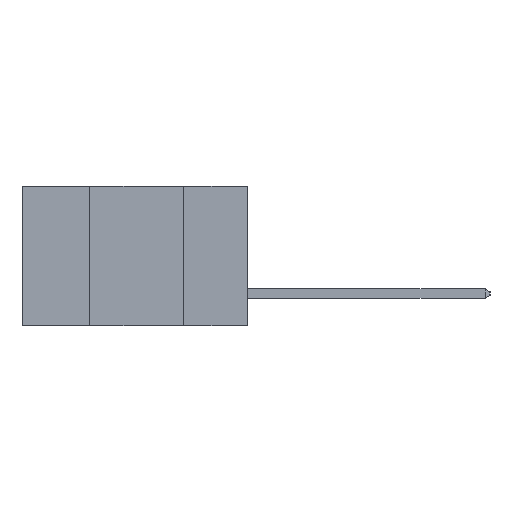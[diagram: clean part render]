
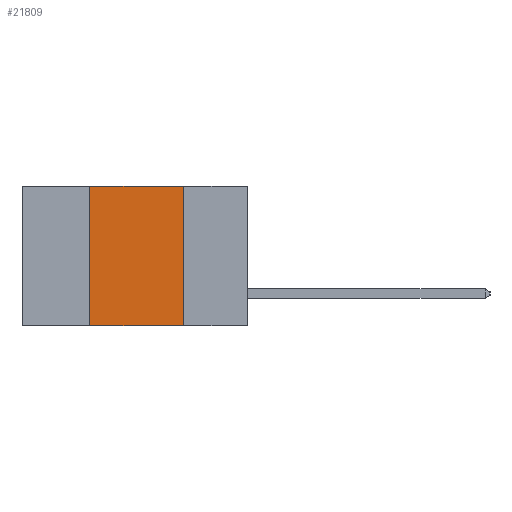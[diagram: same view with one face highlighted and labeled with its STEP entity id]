
A CAD part, left-side view. The second image highlights one B-rep face of the part: STEP entity #21809.
In plain terms, the highlighted planar face has unit normal (-1, 0, 0).
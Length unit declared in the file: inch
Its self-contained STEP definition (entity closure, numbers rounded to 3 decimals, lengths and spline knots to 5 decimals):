
#1304 = CARTESIAN_POINT ( 'NONE',  ( 0., 0.42, -0.37 ) ) ;
#1460 = CARTESIAN_POINT ( 'NONE',  ( 0., 0.17, 0. ) ) ;
#2039 = EDGE_CURVE ( 'NONE', #16251, #20413, #9631, .T. ) ;
#2403 = CARTESIAN_POINT ( 'NONE',  ( 0., 0.42, 0. ) ) ;
#2619 = CARTESIAN_POINT ( 'NONE',  ( 0., 0.6, 0. ) ) ;
#2816 = CARTESIAN_POINT ( 'NONE',  ( 0., 0.42, 0. ) ) ;
#4163 = VECTOR ( 'NONE', #11930, 39.37008 ) ;
#4676 = DIRECTION ( 'NONE',  ( 1., 0., 0. ) ) ;
#5039 = VERTEX_POINT ( 'NONE', #1304 ) ;
#5864 = LINE ( 'NONE', #18044, #25113 ) ;
#5946 = EDGE_CURVE ( 'NONE', #20413, #9562, #23006, .T. ) ;
#6793 = ORIENTED_EDGE ( 'NONE', *, *, #18635, .F. ) ;
#6980 = CARTESIAN_POINT ( 'NONE',  ( 0., 0.17, -0.37 ) ) ;
#6997 = DIRECTION ( 'NONE',  ( 0., 0., -1. ) ) ;
#8268 = AXIS2_PLACEMENT_3D ( 'NONE', #2619, #4676, #18788 ) ;
#9192 = EDGE_LOOP ( 'NONE', ( #21666, #16491, #6793, #16978 ) ) ;
#9562 = VERTEX_POINT ( 'NONE', #6980 ) ;
#9631 = LINE ( 'NONE', #11522, #4163 ) ;
#11522 = CARTESIAN_POINT ( 'NONE',  ( 0., 0.6, 0. ) ) ;
#11930 = DIRECTION ( 'NONE',  ( 0., -1., 0. ) ) ;
#13063 = LINE ( 'NONE', #2403, #18353 ) ;
#14804 = PLANE ( 'NONE',  #8268 ) ;
#15982 = EDGE_CURVE ( 'NONE', #5039, #9562, #5864, .T. ) ;
#16251 = VERTEX_POINT ( 'NONE', #2816 ) ;
#16491 = ORIENTED_EDGE ( 'NONE', *, *, #2039, .F. ) ;
#16978 = ORIENTED_EDGE ( 'NONE', *, *, #15982, .T. ) ;
#17901 = VECTOR ( 'NONE', #6997, 39.37008 ) ;
#18044 = CARTESIAN_POINT ( 'NONE',  ( 0., 0.6, -0.37 ) ) ;
#18353 = VECTOR ( 'NONE', #18584, 39.37008 ) ;
#18584 = DIRECTION ( 'NONE',  ( 0., 0., 1. ) ) ;
#18635 = EDGE_CURVE ( 'NONE', #5039, #16251, #13063, .T. ) ;
#18788 = DIRECTION ( 'NONE',  ( 0., 0., -1. ) ) ;
#19467 = FACE_OUTER_BOUND ( 'NONE', #9192, .T. ) ;
#20413 = VERTEX_POINT ( 'NONE', #22036 ) ;
#21666 = ORIENTED_EDGE ( 'NONE', *, *, #5946, .F. ) ;
#21809 = ADVANCED_FACE ( 'NONE', ( #19467 ), #14804, .F. ) ;
#22036 = CARTESIAN_POINT ( 'NONE',  ( 0., 0.17, 0. ) ) ;
#23006 = LINE ( 'NONE', #1460, #17901 ) ;
#23829 = DIRECTION ( 'NONE',  ( 0., -1., 0. ) ) ;
#25113 = VECTOR ( 'NONE', #23829, 39.37008 ) ;
